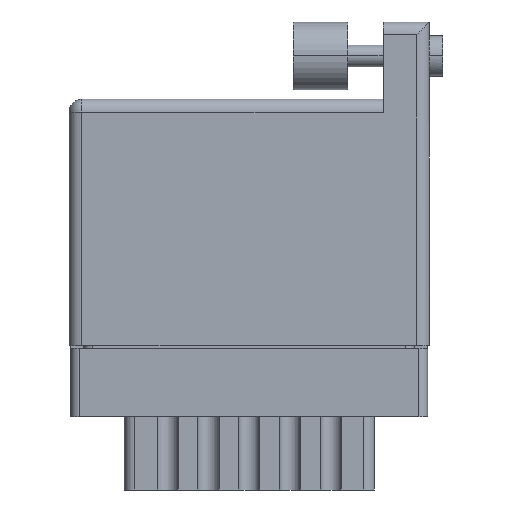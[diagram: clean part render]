
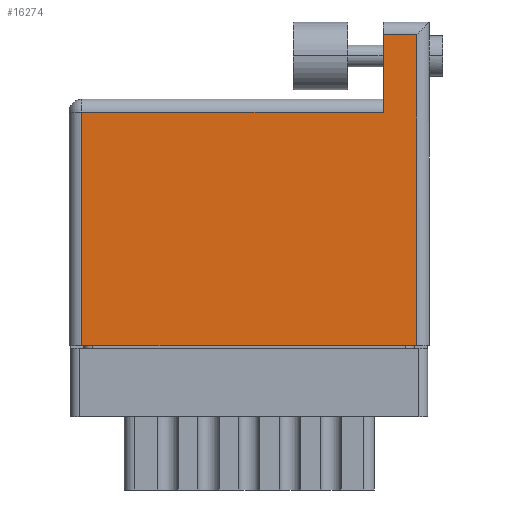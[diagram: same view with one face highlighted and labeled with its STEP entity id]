
A CAD part, front view. The second image highlights one B-rep face of the part: STEP entity #16274.
In plain terms, the highlighted face is planar.
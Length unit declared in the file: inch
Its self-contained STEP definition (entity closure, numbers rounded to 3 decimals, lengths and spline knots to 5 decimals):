
#366 = PLANE ( 'NONE',  #25162 ) ;
#598 = LINE ( 'NONE', #10863, #4022 ) ;
#1927 = DIRECTION ( 'NONE',  ( -1., 0., 0. ) ) ;
#2209 = CARTESIAN_POINT ( 'NONE',  ( 1.155, 1.143, 0. ) ) ;
#2646 = CARTESIAN_POINT ( 'NONE',  ( 1.278, 1.19, 0. ) ) ;
#3340 = EDGE_CURVE ( 'NONE', #15610, #23334, #10003, .T. ) ;
#3596 = FACE_OUTER_BOUND ( 'NONE', #20913, .T. ) ;
#4022 = VECTOR ( 'NONE', #7007, 39.37008 ) ;
#5072 = DIRECTION ( 'NONE',  ( -1., 0., 0. ) ) ;
#5743 = LINE ( 'NONE', #20478, #13581 ) ;
#5767 = EDGE_CURVE ( 'NONE', #19454, #15610, #12087, .T. ) ;
#6213 = DIRECTION ( 'NONE',  ( 0., 0., -1. ) ) ;
#6758 = VECTOR ( 'NONE', #1927, 39.37008 ) ;
#6922 = ORIENTED_EDGE ( 'NONE', *, *, #5767, .T. ) ;
#6953 = ORIENTED_EDGE ( 'NONE', *, *, #3340, .T. ) ;
#7002 = CARTESIAN_POINT ( 'NONE',  ( 1.155, 1.143, 0. ) ) ;
#7007 = DIRECTION ( 'NONE',  ( 1., 0., 0. ) ) ;
#7769 = CARTESIAN_POINT ( 'NONE',  ( 0., 0.859, 0. ) ) ;
#8277 = LINE ( 'NONE', #2646, #12354 ) ;
#9557 = VERTEX_POINT ( 'NONE', #16622 ) ;
#9833 = EDGE_CURVE ( 'NONE', #23334, #20802, #598, .T. ) ;
#10003 = LINE ( 'NONE', #20403, #23525 ) ;
#10863 = CARTESIAN_POINT ( 'NONE',  ( 0., 0., 0. ) ) ;
#11640 = EDGE_CURVE ( 'NONE', #9557, #15219, #14918, .T. ) ;
#12087 = LINE ( 'NONE', #7769, #6758 ) ;
#12354 = VECTOR ( 'NONE', #25094, 39.37008 ) ;
#12371 = CARTESIAN_POINT ( 'NONE',  ( 1.278, 0., 0. ) ) ;
#13556 = ORIENTED_EDGE ( 'NONE', *, *, #11640, .T. ) ;
#13581 = VECTOR ( 'NONE', #14667, 39.37008 ) ;
#14071 = ORIENTED_EDGE ( 'NONE', *, *, #9833, .T. ) ;
#14321 = ORIENTED_EDGE ( 'NONE', *, *, #16438, .T. ) ;
#14667 = DIRECTION ( 'NONE',  ( 0., -1., 0. ) ) ;
#14918 = LINE ( 'NONE', #7002, #19613 ) ;
#15219 = VERTEX_POINT ( 'NONE', #2209 ) ;
#15610 = VERTEX_POINT ( 'NONE', #22330 ) ;
#16274 = ADVANCED_FACE ( 'NONE', ( #3596 ), #366, .F. ) ;
#16438 = EDGE_CURVE ( 'NONE', #20802, #9557, #8277, .T. ) ;
#16565 = CARTESIAN_POINT ( 'NONE',  ( 0., 0.906, 0. ) ) ;
#16622 = CARTESIAN_POINT ( 'NONE',  ( 1.278, 1.143, 0. ) ) ;
#17508 = CARTESIAN_POINT ( 'NONE',  ( 0.047, 0., 0. ) ) ;
#19134 = EDGE_CURVE ( 'NONE', #15219, #19454, #5743, .T. ) ;
#19454 = VERTEX_POINT ( 'NONE', #25463 ) ;
#19613 = VECTOR ( 'NONE', #5072, 39.37008 ) ;
#20403 = CARTESIAN_POINT ( 'NONE',  ( 0.047, 0., 0. ) ) ;
#20478 = CARTESIAN_POINT ( 'NONE',  ( 1.155, 1.19, 0. ) ) ;
#20637 = DIRECTION ( 'NONE',  ( -1., 0., 0. ) ) ;
#20802 = VERTEX_POINT ( 'NONE', #12371 ) ;
#20913 = EDGE_LOOP ( 'NONE', ( #14071, #14321, #13556, #23720, #6922, #6953 ) ) ;
#22330 = CARTESIAN_POINT ( 'NONE',  ( 0.047, 0.859, 0. ) ) ;
#23334 = VERTEX_POINT ( 'NONE', #17508 ) ;
#23525 = VECTOR ( 'NONE', #24609, 39.37008 ) ;
#23720 = ORIENTED_EDGE ( 'NONE', *, *, #19134, .T. ) ;
#24609 = DIRECTION ( 'NONE',  ( 0., -1., 0. ) ) ;
#25094 = DIRECTION ( 'NONE',  ( 0., 1., 0. ) ) ;
#25162 = AXIS2_PLACEMENT_3D ( 'NONE', #16565, #6213, #20637 ) ;
#25463 = CARTESIAN_POINT ( 'NONE',  ( 1.155, 0.859, 0. ) ) ;
